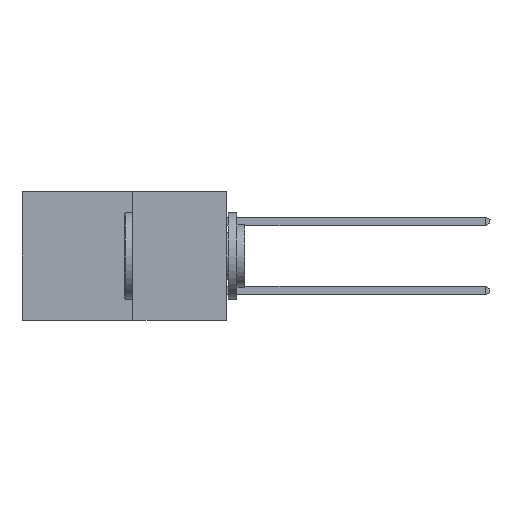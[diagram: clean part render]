
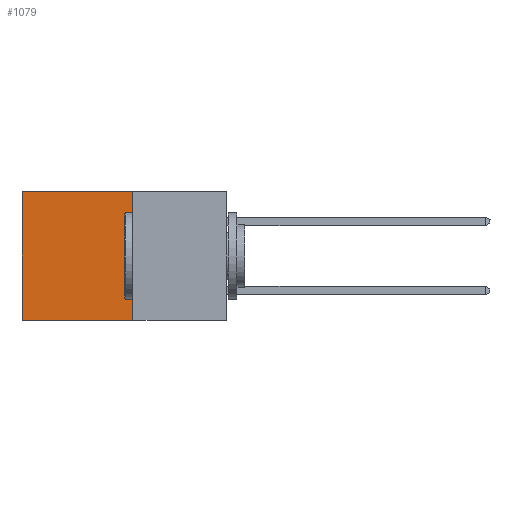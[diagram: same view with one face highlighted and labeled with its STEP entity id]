
A CAD part, left-side view. The second image highlights one B-rep face of the part: STEP entity #1079.
In plain terms, the highlighted planar face has unit normal (-1, 0, 0).
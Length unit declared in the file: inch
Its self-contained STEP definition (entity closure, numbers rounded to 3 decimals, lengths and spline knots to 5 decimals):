
#999 = EDGE_LOOP ( 'NONE', ( #6793, #6727, #4283, #8919 ) ) ;
#1004 = FACE_OUTER_BOUND ( 'NONE', #999, .T. ) ;
#1079 = ADVANCED_FACE ( 'NONE', ( #1004 ), #10017, .F. ) ;
#1396 = EDGE_CURVE ( 'NONE', #8913, #9685, #1973, .T. ) ;
#1897 = CARTESIAN_POINT ( 'NONE',  ( 0.277, 0.27, -0.37 ) ) ;
#1973 = LINE ( 'NONE', #3723, #6720 ) ;
#2370 = EDGE_CURVE ( 'NONE', #11638, #3034, #7675, .T. ) ;
#2416 = VECTOR ( 'NONE', #11477, 39.37008 ) ;
#2943 = CARTESIAN_POINT ( 'NONE',  ( 0.277, 0.59, -0.37 ) ) ;
#3034 = VERTEX_POINT ( 'NONE', #2943 ) ;
#3612 = DIRECTION ( 'NONE',  ( 0., 0., -1. ) ) ;
#3666 = LINE ( 'NONE', #10218, #10494 ) ;
#3723 = CARTESIAN_POINT ( 'NONE',  ( 0.277, 0.27, -0.37 ) ) ;
#4283 = ORIENTED_EDGE ( 'NONE', *, *, #1396, .F. ) ;
#6210 = CARTESIAN_POINT ( 'NONE',  ( 0.277, 0.59, 0. ) ) ;
#6257 = AXIS2_PLACEMENT_3D ( 'NONE', #10155, #9961, #9959 ) ;
#6402 = CARTESIAN_POINT ( 'NONE',  ( 0.277, 0.27, -0.37 ) ) ;
#6720 = VECTOR ( 'NONE', #3612, 39.37008 ) ;
#6727 = ORIENTED_EDGE ( 'NONE', *, *, #10942, .F. ) ;
#6793 = ORIENTED_EDGE ( 'NONE', *, *, #2370, .T. ) ;
#6865 = DIRECTION ( 'NONE',  ( 0., 1., 0. ) ) ;
#7675 = LINE ( 'NONE', #11706, #2416 ) ;
#8184 = CARTESIAN_POINT ( 'NONE',  ( 0.277, 0.27, 0. ) ) ;
#8336 = EDGE_CURVE ( 'NONE', #8913, #11638, #3666, .T. ) ;
#8913 = VERTEX_POINT ( 'NONE', #8184 ) ;
#8919 = ORIENTED_EDGE ( 'NONE', *, *, #8336, .T. ) ;
#9282 = VECTOR ( 'NONE', #10903, 39.37008 ) ;
#9685 = VERTEX_POINT ( 'NONE', #6402 ) ;
#9959 = DIRECTION ( 'NONE',  ( 0., 0., -1. ) ) ;
#9961 = DIRECTION ( 'NONE',  ( 1., 0., 0. ) ) ;
#10017 = PLANE ( 'NONE',  #6257 ) ;
#10155 = CARTESIAN_POINT ( 'NONE',  ( 0.277, 0.27, -0.37 ) ) ;
#10218 = CARTESIAN_POINT ( 'NONE',  ( 0.277, 0.27, 0. ) ) ;
#10494 = VECTOR ( 'NONE', #6865, 39.37008 ) ;
#10903 = DIRECTION ( 'NONE',  ( 0., 1., 0. ) ) ;
#10942 = EDGE_CURVE ( 'NONE', #9685, #3034, #11472, .T. ) ;
#11472 = LINE ( 'NONE', #1897, #9282 ) ;
#11477 = DIRECTION ( 'NONE',  ( 0., 0., -1. ) ) ;
#11638 = VERTEX_POINT ( 'NONE', #6210 ) ;
#11706 = CARTESIAN_POINT ( 'NONE',  ( 0.277, 0.59, -0.37 ) ) ;
